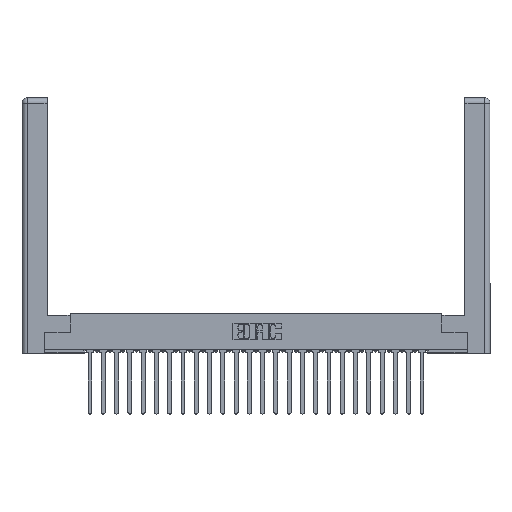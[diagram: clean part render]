
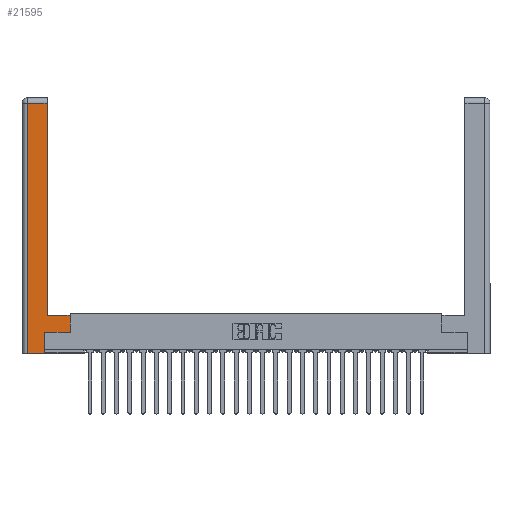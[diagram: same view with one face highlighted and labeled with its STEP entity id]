
A CAD part, top view. The second image highlights one B-rep face of the part: STEP entity #21595.
In plain terms, the highlighted planar face has unit normal (0, 0, 1).
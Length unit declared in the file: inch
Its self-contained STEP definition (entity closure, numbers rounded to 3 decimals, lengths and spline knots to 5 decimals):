
#216 = VERTEX_POINT ( 'NONE', #21365 ) ;
#1174 = CARTESIAN_POINT ( 'NONE',  ( 0.565, 0.245, 0. ) ) ;
#1259 = DIRECTION ( 'NONE',  ( -1., 0., 0. ) ) ;
#1643 = LINE ( 'NONE', #7532, #5847 ) ;
#2436 = CARTESIAN_POINT ( 'NONE',  ( 0.295, 2.94, 0. ) ) ;
#2443 = ORIENTED_EDGE ( 'NONE', *, *, #23491, .T. ) ;
#2609 = VERTEX_POINT ( 'NONE', #14079 ) ;
#2830 = LINE ( 'NONE', #21579, #26346 ) ;
#2956 = EDGE_CURVE ( 'NONE', #11925, #216, #5753, .T. ) ;
#3161 = DIRECTION ( 'NONE',  ( 0., 0., -1. ) ) ;
#3295 = DIRECTION ( 'NONE',  ( 0., 1., 0. ) ) ;
#3380 = VERTEX_POINT ( 'NONE', #9274 ) ;
#3565 = VERTEX_POINT ( 'NONE', #2436 ) ;
#3748 = CARTESIAN_POINT ( 'NONE',  ( 0.265, 0., 0. ) ) ;
#3942 = VECTOR ( 'NONE', #14109, 39.37008 ) ;
#4489 = ORIENTED_EDGE ( 'NONE', *, *, #9974, .T. ) ;
#5380 = ORIENTED_EDGE ( 'NONE', *, *, #15328, .T. ) ;
#5472 = VERTEX_POINT ( 'NONE', #1174 ) ;
#5753 = LINE ( 'NONE', #20008, #14063 ) ;
#5847 = VECTOR ( 'NONE', #1259, 39.37008 ) ;
#6362 = CARTESIAN_POINT ( 'NONE',  ( 0.565, 0.245, 0. ) ) ;
#6802 = LINE ( 'NONE', #25410, #18260 ) ;
#7532 = CARTESIAN_POINT ( 'NONE',  ( 0.0615, 2.94, 0. ) ) ;
#8770 = ORIENTED_EDGE ( 'NONE', *, *, #12814, .T. ) ;
#9202 = DIRECTION ( 'NONE',  ( 0., -1., 0. ) ) ;
#9274 = CARTESIAN_POINT ( 'NONE',  ( 0.0615, 0., 0. ) ) ;
#9426 = CARTESIAN_POINT ( 'NONE',  ( 0., 0., 0. ) ) ;
#9677 = FACE_OUTER_BOUND ( 'NONE', #14147, .T. ) ;
#9817 = CARTESIAN_POINT ( 'NONE',  ( 0.295, 3., 0. ) ) ;
#9974 = EDGE_CURVE ( 'NONE', #3380, #23437, #6802, .T. ) ;
#11925 = VERTEX_POINT ( 'NONE', #25610 ) ;
#11939 = CARTESIAN_POINT ( 'NONE',  ( 0.565, 0.45, 0. ) ) ;
#11948 = ORIENTED_EDGE ( 'NONE', *, *, #2956, .T. ) ;
#12667 = ORIENTED_EDGE ( 'NONE', *, *, #15331, .T. ) ;
#12814 = EDGE_CURVE ( 'NONE', #13661, #3380, #25381, .T. ) ;
#13024 = AXIS2_PLACEMENT_3D ( 'NONE', #9426, #3161, #15671 ) ;
#13238 = CARTESIAN_POINT ( 'NONE',  ( 0.0615, 2.94, 0. ) ) ;
#13661 = VERTEX_POINT ( 'NONE', #13238 ) ;
#14063 = VECTOR ( 'NONE', #22040, 39.37008 ) ;
#14079 = CARTESIAN_POINT ( 'NONE',  ( 0.265, 0.245, 0. ) ) ;
#14109 = DIRECTION ( 'NONE',  ( 0., 1., 0. ) ) ;
#14147 = EDGE_LOOP ( 'NONE', ( #5380, #12667, #8770, #4489, #24181, #25841, #2443, #11948 ) ) ;
#14657 = DIRECTION ( 'NONE',  ( 1., 0., 0. ) ) ;
#15328 = EDGE_CURVE ( 'NONE', #216, #3565, #22299, .T. ) ;
#15331 = EDGE_CURVE ( 'NONE', #3565, #13661, #1643, .T. ) ;
#15671 = DIRECTION ( 'NONE',  ( -1., 0., 0. ) ) ;
#17332 = CARTESIAN_POINT ( 'NONE',  ( 0.0615, 0., 0. ) ) ;
#17367 = EDGE_CURVE ( 'NONE', #23437, #2609, #2830, .T. ) ;
#17557 = VECTOR ( 'NONE', #3295, 39.37008 ) ;
#18260 = VECTOR ( 'NONE', #23629, 39.37008 ) ;
#19008 = DIRECTION ( 'NONE',  ( 0., 1., 0. ) ) ;
#19745 = PLANE ( 'NONE',  #13024 ) ;
#20008 = CARTESIAN_POINT ( 'NONE',  ( 0.295, 0.45, 0. ) ) ;
#20744 = LINE ( 'NONE', #6362, #25726 ) ;
#21365 = CARTESIAN_POINT ( 'NONE',  ( 0.295, 0.45, 0. ) ) ;
#21579 = CARTESIAN_POINT ( 'NONE',  ( 0.265, 0.245, 0. ) ) ;
#21595 = ADVANCED_FACE ( 'NONE', ( #9677 ), #19745, .F. ) ;
#22040 = DIRECTION ( 'NONE',  ( -1., 0., 0. ) ) ;
#22299 = LINE ( 'NONE', #9817, #17557 ) ;
#23437 = VERTEX_POINT ( 'NONE', #3748 ) ;
#23491 = EDGE_CURVE ( 'NONE', #5472, #11925, #24427, .T. ) ;
#23533 = VECTOR ( 'NONE', #9202, 39.37008 ) ;
#23629 = DIRECTION ( 'NONE',  ( 1., 0., 0. ) ) ;
#24181 = ORIENTED_EDGE ( 'NONE', *, *, #17367, .T. ) ;
#24427 = LINE ( 'NONE', #11939, #3942 ) ;
#25381 = LINE ( 'NONE', #17332, #23533 ) ;
#25410 = CARTESIAN_POINT ( 'NONE',  ( 0.265, 0., 0. ) ) ;
#25610 = CARTESIAN_POINT ( 'NONE',  ( 0.565, 0.45, 0. ) ) ;
#25726 = VECTOR ( 'NONE', #14657, 39.37008 ) ;
#25841 = ORIENTED_EDGE ( 'NONE', *, *, #26416, .T. ) ;
#26346 = VECTOR ( 'NONE', #19008, 39.37008 ) ;
#26416 = EDGE_CURVE ( 'NONE', #2609, #5472, #20744, .T. ) ;
